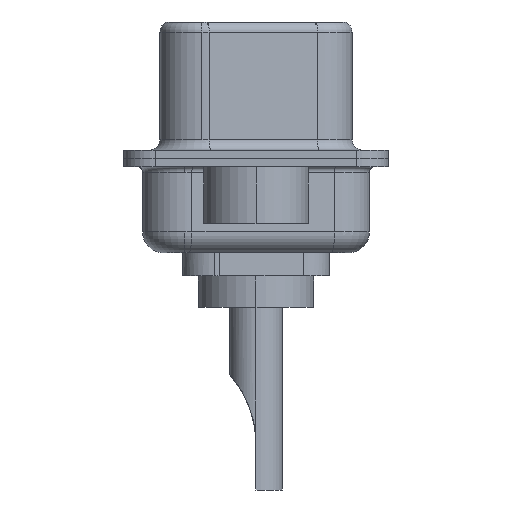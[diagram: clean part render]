
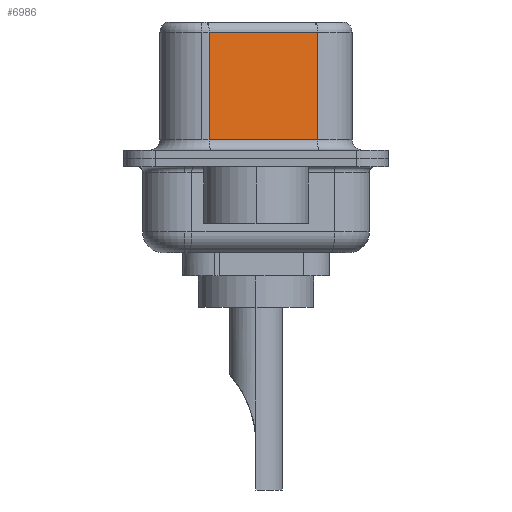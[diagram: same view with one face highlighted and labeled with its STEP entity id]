
A CAD part, left-side view. The second image highlights one B-rep face of the part: STEP entity #6986.
In plain terms, the highlighted planar face has unit normal (-0.985, -0.174, 0).
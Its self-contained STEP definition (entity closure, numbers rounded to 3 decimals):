
#253 = VERTEX_POINT ( 'NONE', #1463 ) ;
#549 = FACE_OUTER_BOUND ( 'NONE', #13410, .T. ) ;
#1281 = CARTESIAN_POINT ( 'NONE',  ( 4.58, -2.927, 6.52 ) ) ;
#1463 = CARTESIAN_POINT ( 'NONE',  ( 4.58, -2.927, 6.02 ) ) ;
#1906 = VERTEX_POINT ( 'NONE', #15966 ) ;
#2691 = CARTESIAN_POINT ( 'NONE',  ( 3.67, 2.233, 0.9 ) ) ;
#4188 = DIRECTION ( 'NONE',  ( 0., 0., -1. ) ) ;
#4915 = LINE ( 'NONE', #8617, #7432 ) ;
#6215 = DIRECTION ( 'NONE',  ( -0.174, 0.985, 0. ) ) ;
#6986 = ADVANCED_FACE ( 'NONE', ( #549 ), #17378, .F. ) ;
#6992 = VERTEX_POINT ( 'NONE', #2691 ) ;
#7211 = VECTOR ( 'NONE', #6215, 1000. ) ;
#7244 = AXIS2_PLACEMENT_3D ( 'NONE', #1281, #14500, #8688 ) ;
#7432 = VECTOR ( 'NONE', #4188, 1000. ) ;
#7819 = CARTESIAN_POINT ( 'NONE',  ( 4.58, -2.927, 0.9 ) ) ;
#8617 = CARTESIAN_POINT ( 'NONE',  ( 4.58, -2.927, 6.52 ) ) ;
#8655 = LINE ( 'NONE', #7819, #13006 ) ;
#8688 = DIRECTION ( 'NONE',  ( -0.174, 0.985, 0. ) ) ;
#8857 = VECTOR ( 'NONE', #12982, 1000. ) ;
#9723 = LINE ( 'NONE', #13612, #7211 ) ;
#10604 = ORIENTED_EDGE ( 'NONE', *, *, #14906, .T. ) ;
#11158 = LINE ( 'NONE', #17439, #8857 ) ;
#11420 = CARTESIAN_POINT ( 'NONE',  ( 3.67, 2.233, 6.02 ) ) ;
#11501 = ORIENTED_EDGE ( 'NONE', *, *, #14433, .T. ) ;
#12546 = ORIENTED_EDGE ( 'NONE', *, *, #17935, .T. ) ;
#12982 = DIRECTION ( 'NONE',  ( 0., 0., -1. ) ) ;
#13006 = VECTOR ( 'NONE', #15797, 1000. ) ;
#13410 = EDGE_LOOP ( 'NONE', ( #13826, #12546, #11501, #10604 ) ) ;
#13612 = CARTESIAN_POINT ( 'NONE',  ( 4.58, -2.927, 6.02 ) ) ;
#13826 = ORIENTED_EDGE ( 'NONE', *, *, #18294, .F. ) ;
#14103 = VERTEX_POINT ( 'NONE', #11420 ) ;
#14433 = EDGE_CURVE ( 'NONE', #14103, #6992, #11158, .T. ) ;
#14500 = DIRECTION ( 'NONE',  ( 0.985, 0.174, 0. ) ) ;
#14906 = EDGE_CURVE ( 'NONE', #6992, #1906, #8655, .T. ) ;
#15797 = DIRECTION ( 'NONE',  ( 0.174, -0.985, 0. ) ) ;
#15966 = CARTESIAN_POINT ( 'NONE',  ( 4.58, -2.927, 0.9 ) ) ;
#17378 = PLANE ( 'NONE',  #7244 ) ;
#17439 = CARTESIAN_POINT ( 'NONE',  ( 3.67, 2.233, 6.52 ) ) ;
#17935 = EDGE_CURVE ( 'NONE', #253, #14103, #9723, .T. ) ;
#18294 = EDGE_CURVE ( 'NONE', #253, #1906, #4915, .T. ) ;
